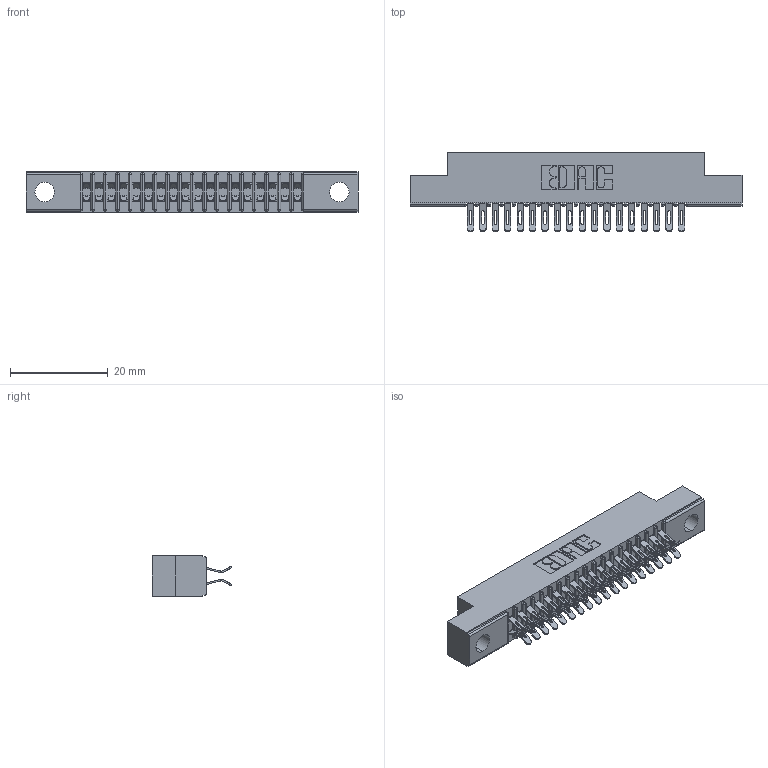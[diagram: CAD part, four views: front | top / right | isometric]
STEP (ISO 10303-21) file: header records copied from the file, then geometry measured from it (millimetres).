
FILE_DESCRIPTION (( 'STEP AP203' ), '1' );
FILE_NAME ('391-036-555-204.STEP', '2018-08-08T23:38:10', ( '' ), ( '' ), 'SwSTEP 2.0', 'SolidWorks 2016', '' );
FILE_SCHEMA (( 'CONFIG_CONTROL_DESIGN' ));
Length unit declared in the file: inch
Products named in the file (3): 341-292-001_341-292-155; 391-036-555-204; 341 Part_.156 (3.96) Dia Mounting Holes
Assembly tree (37 placements, depth 2):
  391-036-555-204
    341 Part_.156 (3.96) Dia Mounting Holes
    341-292-001_341-292-155  x36
Bounding box: 67.94 x 16.31 x 8.38 mm (x, y, z)
Volume: 3818.9 mm3; surface area: 7906.3 mm2
Topology: 37 solids, 37 shells, 2938 faces, 8758 edges, 5702 vertices
Faces by surface type: plane 1594, cylinder 1272, sphere 38, torus 34
Entity records: 25869 total; most frequent: CARTESIAN_POINT 4322, ORIENTED_EDGE 4280, DIRECTION 4194, EDGE_CURVE 2140, LINE 1694, VECTOR 1694, VERTEX_POINT 1362, AXIS2_PLACEMENT_3D 1250
